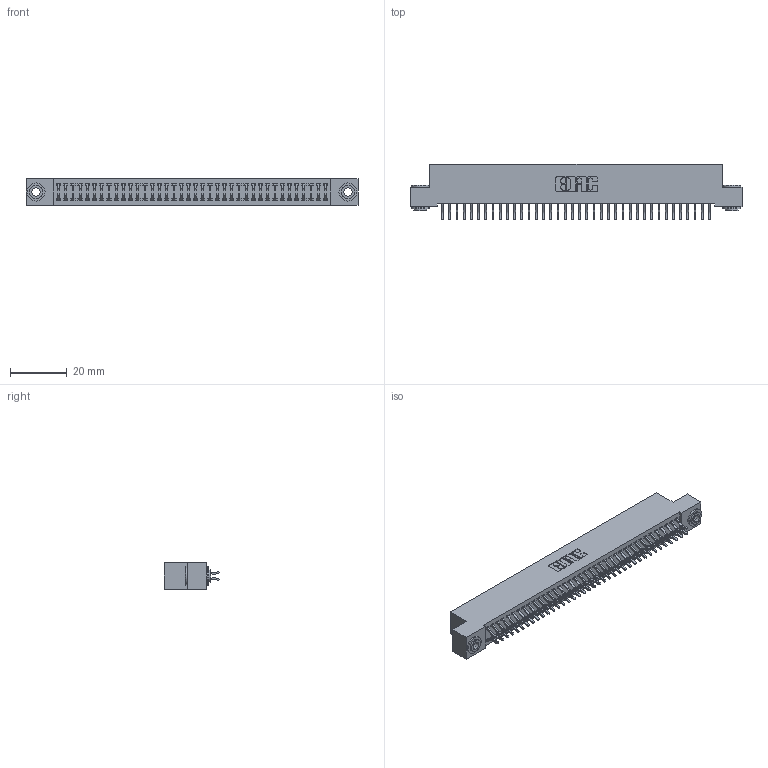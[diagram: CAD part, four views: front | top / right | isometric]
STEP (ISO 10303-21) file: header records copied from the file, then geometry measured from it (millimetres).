
FILE_DESCRIPTION (( 'STEP AP203' ), '1' );
FILE_NAME ('342-076-556-203.STEP', '2019-10-04T10:52:03', ( '' ), ( '' ), 'SwSTEP 2.0', 'SolidWorks 2016', '' );
FILE_SCHEMA (( 'CONFIG_CONTROL_DESIGN' ));
Length unit declared in the file: inch
Products named in the file (4): 342 Part_.156 TH; 345-292-001_556 Tail; 342-250-002_345-250-002-102; 342-076-556-203
Assembly tree (79 placements, depth 2):
  342-076-556-203
    342 Part_.156 TH
    345-292-001_556 Tail  x76
    342-250-002_345-250-002-102  x2
Bounding box: 116.84 x 19.58 x 9.4 mm (x, y, z)
Volume: 10500 mm3; surface area: 17133.2 mm2
Topology: 79 solids, 79 shells, 4556 faces, 13523 edges, 8910 vertices
Faces by surface type: plane 3116, cylinder 1432, cone 8
Entity records: 25702 total; most frequent: CARTESIAN_POINT 4253, ORIENTED_EDGE 4170, DIRECTION 3663, EDGE_CURVE 2085, LINE 1925, VECTOR 1925, VERTEX_POINT 1386, AXIS2_PLACEMENT_3D 869
